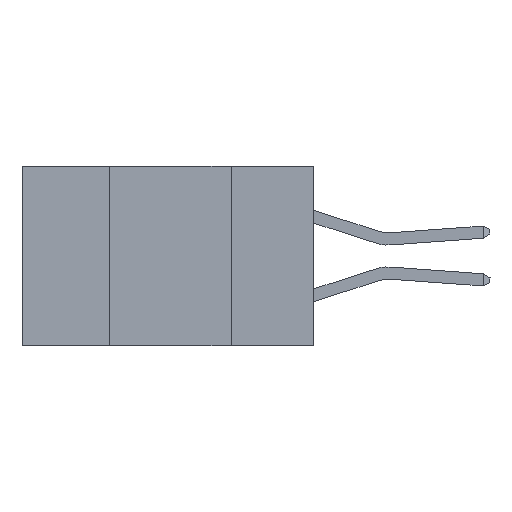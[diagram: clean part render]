
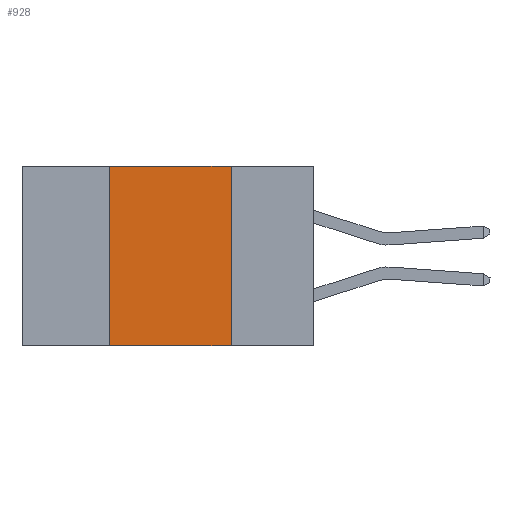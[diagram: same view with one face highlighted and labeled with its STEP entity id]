
A CAD part, left-side view. The second image highlights one B-rep face of the part: STEP entity #928.
In plain terms, the highlighted planar face has unit normal (-1, 0, 0).
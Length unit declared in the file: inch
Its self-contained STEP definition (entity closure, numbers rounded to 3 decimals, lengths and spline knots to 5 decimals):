
#464 = EDGE_CURVE ( 'NONE', #3547, #8521, #11679, .T. ) ;
#928 = ADVANCED_FACE ( 'NONE', ( #17394 ), #8963, .F. ) ;
#1157 = LINE ( 'NONE', #8208, #15517 ) ;
#1199 = CARTESIAN_POINT ( 'NONE',  ( 0., 0.17, 0. ) ) ;
#2326 = VECTOR ( 'NONE', #17295, 39.37008 ) ;
#3547 = VERTEX_POINT ( 'NONE', #9698 ) ;
#3566 = DIRECTION ( 'NONE',  ( 1., 0., 0. ) ) ;
#4113 = CARTESIAN_POINT ( 'NONE',  ( 0., 0.17, 0. ) ) ;
#4115 = VERTEX_POINT ( 'NONE', #19228 ) ;
#5528 = VERTEX_POINT ( 'NONE', #1199 ) ;
#6646 = ORIENTED_EDGE ( 'NONE', *, *, #464, .T. ) ;
#8082 = ORIENTED_EDGE ( 'NONE', *, *, #20527, .F. ) ;
#8208 = CARTESIAN_POINT ( 'NONE',  ( 0., 0.42, 0. ) ) ;
#8521 = VERTEX_POINT ( 'NONE', #12342 ) ;
#8610 = EDGE_CURVE ( 'NONE', #5528, #8521, #19278, .T. ) ;
#8674 = DIRECTION ( 'NONE',  ( 0., 0., -1. ) ) ;
#8963 = PLANE ( 'NONE',  #19462 ) ;
#9597 = DIRECTION ( 'NONE',  ( 0., -1., 0. ) ) ;
#9622 = DIRECTION ( 'NONE',  ( 0., -1., 0. ) ) ;
#9698 = CARTESIAN_POINT ( 'NONE',  ( 0., 0.42, -0.37 ) ) ;
#10980 = ORIENTED_EDGE ( 'NONE', *, *, #21196, .F. ) ;
#11679 = LINE ( 'NONE', #19846, #19986 ) ;
#12342 = CARTESIAN_POINT ( 'NONE',  ( 0., 0.17, -0.37 ) ) ;
#12768 = CARTESIAN_POINT ( 'NONE',  ( 0., 0.6, 0. ) ) ;
#14574 = CARTESIAN_POINT ( 'NONE',  ( 0., 0.6, 0. ) ) ;
#15322 = ORIENTED_EDGE ( 'NONE', *, *, #8610, .F. ) ;
#15517 = VECTOR ( 'NONE', #18044, 39.37008 ) ;
#17295 = DIRECTION ( 'NONE',  ( 0., 0., -1. ) ) ;
#17394 = FACE_OUTER_BOUND ( 'NONE', #18003, .T. ) ;
#18003 = EDGE_LOOP ( 'NONE', ( #15322, #10980, #8082, #6646 ) ) ;
#18044 = DIRECTION ( 'NONE',  ( 0., 0., 1. ) ) ;
#19148 = LINE ( 'NONE', #14574, #21437 ) ;
#19228 = CARTESIAN_POINT ( 'NONE',  ( 0., 0.42, 0. ) ) ;
#19278 = LINE ( 'NONE', #4113, #2326 ) ;
#19462 = AXIS2_PLACEMENT_3D ( 'NONE', #12768, #3566, #8674 ) ;
#19846 = CARTESIAN_POINT ( 'NONE',  ( 0., 0.6, -0.37 ) ) ;
#19986 = VECTOR ( 'NONE', #9597, 39.37008 ) ;
#20527 = EDGE_CURVE ( 'NONE', #3547, #4115, #1157, .T. ) ;
#21196 = EDGE_CURVE ( 'NONE', #4115, #5528, #19148, .T. ) ;
#21437 = VECTOR ( 'NONE', #9622, 39.37008 ) ;
